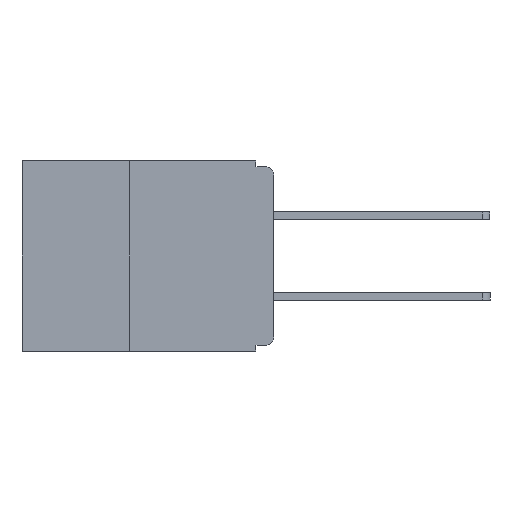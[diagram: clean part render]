
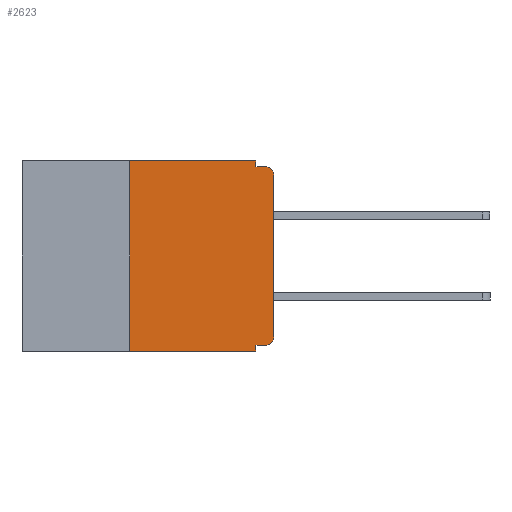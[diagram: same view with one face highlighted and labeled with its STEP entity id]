
A CAD part, left-side view. The second image highlights one B-rep face of the part: STEP entity #2623.
In plain terms, the highlighted planar face has unit normal (-1, 0, 0).
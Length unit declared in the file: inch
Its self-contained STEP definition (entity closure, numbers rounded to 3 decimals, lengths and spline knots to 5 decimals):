
#545 = CARTESIAN_POINT ( 'NONE',  ( 0., 0.437, 0. ) ) ;
#636 = VERTEX_POINT ( 'NONE', #15446 ) ;
#953 = DIRECTION ( 'NONE',  ( 0., 0., -1. ) ) ;
#1400 = VERTEX_POINT ( 'NONE', #17170 ) ;
#1561 = EDGE_CURVE ( 'NONE', #21767, #1400, #27020, .T. ) ;
#2623 = ADVANCED_FACE ( 'NONE', ( #17796 ), #20670, .F. ) ;
#3244 = CARTESIAN_POINT ( 'NONE',  ( 0., 0.015, -0.025 ) ) ;
#3368 = ORIENTED_EDGE ( 'NONE', *, *, #25880, .T. ) ;
#3547 = ORIENTED_EDGE ( 'NONE', *, *, #17098, .T. ) ;
#4321 = CARTESIAN_POINT ( 'NONE',  ( 0., 0., -0.305 ) ) ;
#4398 = EDGE_CURVE ( 'NONE', #4719, #5826, #20833, .T. ) ;
#4408 = CARTESIAN_POINT ( 'NONE',  ( 0., 0.031, -0.33 ) ) ;
#4553 = ORIENTED_EDGE ( 'NONE', *, *, #1561, .F. ) ;
#4719 = VERTEX_POINT ( 'NONE', #6846 ) ;
#4759 = VECTOR ( 'NONE', #18359, 39.37008 ) ;
#4828 = VERTEX_POINT ( 'NONE', #4321 ) ;
#5366 = VECTOR ( 'NONE', #25713, 39.37008 ) ;
#5438 = AXIS2_PLACEMENT_3D ( 'NONE', #3244, #18769, #5526 ) ;
#5526 = DIRECTION ( 'NONE',  ( 0., 0., -1. ) ) ;
#5826 = VERTEX_POINT ( 'NONE', #27676 ) ;
#5828 = CARTESIAN_POINT ( 'NONE',  ( 0., 0.031, 0. ) ) ;
#6182 = ORIENTED_EDGE ( 'NONE', *, *, #13295, .F. ) ;
#6460 = ORIENTED_EDGE ( 'NONE', *, *, #18199, .F. ) ;
#6846 = CARTESIAN_POINT ( 'NONE',  ( 0., 0.015, -0.32 ) ) ;
#7094 = VECTOR ( 'NONE', #26791, 39.37008 ) ;
#7182 = CIRCLE ( 'NONE', #5438, 0.015 ) ;
#7248 = ORIENTED_EDGE ( 'NONE', *, *, #21072, .F. ) ;
#7759 = AXIS2_PLACEMENT_3D ( 'NONE', #27431, #14428, #953 ) ;
#9002 = CARTESIAN_POINT ( 'NONE',  ( 0., 0., 0. ) ) ;
#9535 = CARTESIAN_POINT ( 'NONE',  ( 0., 0.25, -0.33 ) ) ;
#9825 = LINE ( 'NONE', #545, #26571 ) ;
#10516 = ORIENTED_EDGE ( 'NONE', *, *, #27254, .T. ) ;
#10630 = VECTOR ( 'NONE', #24338, 39.37008 ) ;
#10677 = LINE ( 'NONE', #9535, #4759 ) ;
#10727 = CARTESIAN_POINT ( 'NONE',  ( 0., 0.25, -0.33 ) ) ;
#11176 = ORIENTED_EDGE ( 'NONE', *, *, #26256, .F. ) ;
#11328 = LINE ( 'NONE', #9002, #10630 ) ;
#11526 = DIRECTION ( 'NONE',  ( 0., 0., -1. ) ) ;
#11901 = DIRECTION ( 'NONE',  ( 0., -1., 0. ) ) ;
#12984 = LINE ( 'NONE', #15946, #7094 ) ;
#13295 = EDGE_CURVE ( 'NONE', #22733, #21767, #26901, .T. ) ;
#14330 = CIRCLE ( 'NONE', #7759, 0.015 ) ;
#14428 = DIRECTION ( 'NONE',  ( -1., 0., 0. ) ) ;
#14857 = AXIS2_PLACEMENT_3D ( 'NONE', #27018, #24132, #11526 ) ;
#15446 = CARTESIAN_POINT ( 'NONE',  ( 0., 0.25, 0. ) ) ;
#15466 = VECTOR ( 'NONE', #17059, 39.37008 ) ;
#15946 = CARTESIAN_POINT ( 'NONE',  ( 0., 0.437, -0.33 ) ) ;
#16004 = VECTOR ( 'NONE', #25383, 39.37008 ) ;
#16006 = ORIENTED_EDGE ( 'NONE', *, *, #4398, .F. ) ;
#16344 = DIRECTION ( 'NONE',  ( 0., 1., 0. ) ) ;
#16817 = CARTESIAN_POINT ( 'NONE',  ( 0., 0., -0.32 ) ) ;
#17059 = DIRECTION ( 'NONE',  ( 0., -1., 0. ) ) ;
#17098 = EDGE_CURVE ( 'NONE', #18479, #1400, #7182, .T. ) ;
#17170 = CARTESIAN_POINT ( 'NONE',  ( 0., 0.015, -0.01 ) ) ;
#17225 = ORIENTED_EDGE ( 'NONE', *, *, #18268, .T. ) ;
#17722 = EDGE_LOOP ( 'NONE', ( #3368, #3547, #4553, #6182, #6460, #7248, #10516, #11176, #16006, #17225 ) ) ;
#17796 = FACE_OUTER_BOUND ( 'NONE', #17722, .T. ) ;
#18069 = VERTEX_POINT ( 'NONE', #4408 ) ;
#18199 = EDGE_CURVE ( 'NONE', #636, #22733, #9825, .T. ) ;
#18268 = EDGE_CURVE ( 'NONE', #4719, #4828, #14330, .T. ) ;
#18359 = DIRECTION ( 'NONE',  ( 0., 0., 1. ) ) ;
#18479 = VERTEX_POINT ( 'NONE', #23885 ) ;
#18769 = DIRECTION ( 'NONE',  ( -1., 0., 0. ) ) ;
#18822 = CARTESIAN_POINT ( 'NONE',  ( 0., 0.031, 0. ) ) ;
#20670 = PLANE ( 'NONE',  #14857 ) ;
#20833 = LINE ( 'NONE', #16817, #25919 ) ;
#21072 = EDGE_CURVE ( 'NONE', #22206, #636, #10677, .T. ) ;
#21346 = CARTESIAN_POINT ( 'NONE',  ( 0., 0., -0.01 ) ) ;
#21767 = VERTEX_POINT ( 'NONE', #23425 ) ;
#22206 = VERTEX_POINT ( 'NONE', #10727 ) ;
#22733 = VERTEX_POINT ( 'NONE', #5828 ) ;
#22981 = LINE ( 'NONE', #23574, #5366 ) ;
#23425 = CARTESIAN_POINT ( 'NONE',  ( 0., 0.031, -0.01 ) ) ;
#23574 = CARTESIAN_POINT ( 'NONE',  ( 0., 0.031, -0.33 ) ) ;
#23885 = CARTESIAN_POINT ( 'NONE',  ( 0., 0., -0.025 ) ) ;
#24132 = DIRECTION ( 'NONE',  ( 1., 0., 0. ) ) ;
#24338 = DIRECTION ( 'NONE',  ( 0., 0., 1. ) ) ;
#25383 = DIRECTION ( 'NONE',  ( 0., 0., -1. ) ) ;
#25713 = DIRECTION ( 'NONE',  ( 0., 0., -1. ) ) ;
#25880 = EDGE_CURVE ( 'NONE', #4828, #18479, #11328, .T. ) ;
#25919 = VECTOR ( 'NONE', #16344, 39.37008 ) ;
#26256 = EDGE_CURVE ( 'NONE', #5826, #18069, #22981, .T. ) ;
#26571 = VECTOR ( 'NONE', #11901, 39.37008 ) ;
#26791 = DIRECTION ( 'NONE',  ( 0., -1., 0. ) ) ;
#26901 = LINE ( 'NONE', #18822, #16004 ) ;
#27018 = CARTESIAN_POINT ( 'NONE',  ( 0., 0.437, 0. ) ) ;
#27020 = LINE ( 'NONE', #21346, #15466 ) ;
#27254 = EDGE_CURVE ( 'NONE', #22206, #18069, #12984, .T. ) ;
#27431 = CARTESIAN_POINT ( 'NONE',  ( 0., 0.015, -0.305 ) ) ;
#27676 = CARTESIAN_POINT ( 'NONE',  ( 0., 0.031, -0.32 ) ) ;
